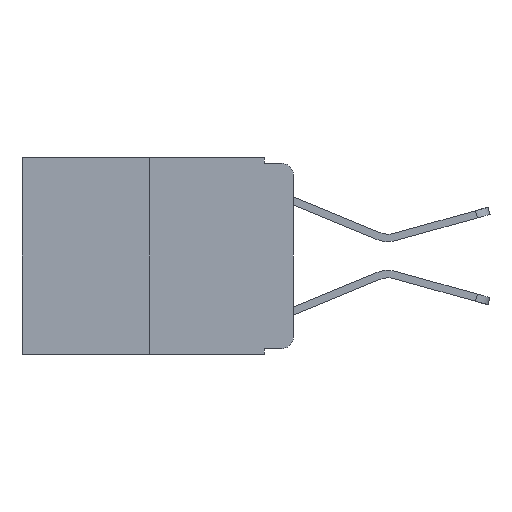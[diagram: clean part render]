
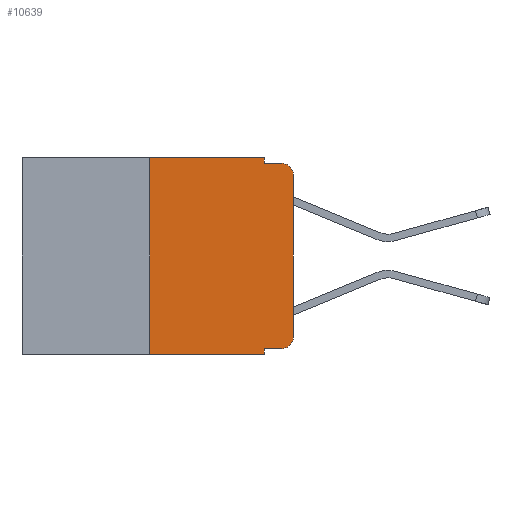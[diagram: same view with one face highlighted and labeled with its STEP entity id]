
A CAD part, left-side view. The second image highlights one B-rep face of the part: STEP entity #10639.
In plain terms, the highlighted planar face has unit normal (-1, 0, 0).
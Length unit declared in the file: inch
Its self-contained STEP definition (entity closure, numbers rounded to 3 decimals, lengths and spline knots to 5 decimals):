
#393 = LINE ( 'NONE', #5756, #20992 ) ;
#685 = DIRECTION ( 'NONE',  ( -1., 0., 0. ) ) ;
#1173 = VERTEX_POINT ( 'NONE', #13284 ) ;
#1434 = CARTESIAN_POINT ( 'NONE',  ( 0., 0.473, -0.343 ) ) ;
#1468 = CARTESIAN_POINT ( 'NONE',  ( 0., 0.25, 0. ) ) ;
#1786 = EDGE_CURVE ( 'NONE', #17790, #16491, #21317, .T. ) ;
#2402 = ORIENTED_EDGE ( 'NONE', *, *, #21774, .F. ) ;
#2690 = EDGE_CURVE ( 'NONE', #3242, #16491, #19737, .T. ) ;
#2977 = EDGE_CURVE ( 'NONE', #11182, #22603, #17582, .T. ) ;
#3242 = VERTEX_POINT ( 'NONE', #4226 ) ;
#3394 = CARTESIAN_POINT ( 'NONE',  ( 0., 0.051, -0.333 ) ) ;
#3872 = VECTOR ( 'NONE', #18371, 39.37008 ) ;
#4160 = AXIS2_PLACEMENT_3D ( 'NONE', #11089, #24662, #13111 ) ;
#4226 = CARTESIAN_POINT ( 'NONE',  ( 0., 0.25, -0.343 ) ) ;
#4704 = ORIENTED_EDGE ( 'NONE', *, *, #12614, .F. ) ;
#4867 = VECTOR ( 'NONE', #12065, 39.37008 ) ;
#4975 = CARTESIAN_POINT ( 'NONE',  ( 0., 0.473, 0. ) ) ;
#5521 = VERTEX_POINT ( 'NONE', #20653 ) ;
#5756 = CARTESIAN_POINT ( 'NONE',  ( 0., 0.051, -0.01 ) ) ;
#5895 = EDGE_CURVE ( 'NONE', #17790, #1173, #25040, .T. ) ;
#5953 = CARTESIAN_POINT ( 'NONE',  ( 0., 0.051, 0. ) ) ;
#6252 = DIRECTION ( 'NONE',  ( 0., -1., 0. ) ) ;
#6632 = EDGE_LOOP ( 'NONE', ( #18409, #18120, #2402, #21161, #15987, #4704, #15985, #20039, #12877, #23218 ) ) ;
#8086 = EDGE_CURVE ( 'NONE', #5521, #17999, #16842, .T. ) ;
#8513 = FACE_OUTER_BOUND ( 'NONE', #6632, .T. ) ;
#9139 = PLANE ( 'NONE',  #23047 ) ;
#9425 = CARTESIAN_POINT ( 'NONE',  ( 0., 0.051, -0.333 ) ) ;
#9535 = VECTOR ( 'NONE', #11433, 39.37008 ) ;
#9882 = DIRECTION ( 'NONE',  ( 0., -1., 0. ) ) ;
#9940 = EDGE_CURVE ( 'NONE', #17999, #14084, #13562, .T. ) ;
#10024 = CARTESIAN_POINT ( 'NONE',  ( 0., 0.051, -0.343 ) ) ;
#10639 = ADVANCED_FACE ( 'NONE', ( #8513 ), #9139, .F. ) ;
#11089 = CARTESIAN_POINT ( 'NONE',  ( 0., 0.02, -0.03 ) ) ;
#11144 = DIRECTION ( 'NONE',  ( 0., 0., -1. ) ) ;
#11182 = VERTEX_POINT ( 'NONE', #24507 ) ;
#11343 = VERTEX_POINT ( 'NONE', #1468 ) ;
#11433 = DIRECTION ( 'NONE',  ( 0., -1., 0. ) ) ;
#11603 = VECTOR ( 'NONE', #24381, 39.37008 ) ;
#11853 = VECTOR ( 'NONE', #14401, 39.37008 ) ;
#12065 = DIRECTION ( 'NONE',  ( 0., 0., -1. ) ) ;
#12128 = EDGE_CURVE ( 'NONE', #1173, #5521, #20756, .T. ) ;
#12212 = CARTESIAN_POINT ( 'NONE',  ( 0., 0., -0.03 ) ) ;
#12381 = VECTOR ( 'NONE', #13945, 39.37008 ) ;
#12614 = EDGE_CURVE ( 'NONE', #3242, #11343, #17082, .T. ) ;
#12788 = CARTESIAN_POINT ( 'NONE',  ( 0., 0.02, -0.313 ) ) ;
#12877 = ORIENTED_EDGE ( 'NONE', *, *, #5895, .T. ) ;
#13111 = DIRECTION ( 'NONE',  ( 0., 0., -1. ) ) ;
#13284 = CARTESIAN_POINT ( 'NONE',  ( 0., 0.02, -0.333 ) ) ;
#13562 = CIRCLE ( 'NONE', #4160, 0.02 ) ;
#13597 = CARTESIAN_POINT ( 'NONE',  ( 0., 0.051, 0. ) ) ;
#13945 = DIRECTION ( 'NONE',  ( 0., 0., -1. ) ) ;
#14084 = VERTEX_POINT ( 'NONE', #15018 ) ;
#14191 = CARTESIAN_POINT ( 'NONE',  ( 0., 0.051, -0.01 ) ) ;
#14401 = DIRECTION ( 'NONE',  ( 0., 0., 1. ) ) ;
#14766 = DIRECTION ( 'NONE',  ( 0., 0., -1. ) ) ;
#14778 = CARTESIAN_POINT ( 'NONE',  ( 0., 0., 0. ) ) ;
#15018 = CARTESIAN_POINT ( 'NONE',  ( 0., 0.02, -0.01 ) ) ;
#15985 = ORIENTED_EDGE ( 'NONE', *, *, #2690, .T. ) ;
#15987 = ORIENTED_EDGE ( 'NONE', *, *, #18081, .F. ) ;
#16491 = VERTEX_POINT ( 'NONE', #10024 ) ;
#16842 = LINE ( 'NONE', #14778, #11603 ) ;
#17082 = LINE ( 'NONE', #22136, #11853 ) ;
#17582 = LINE ( 'NONE', #13597, #12381 ) ;
#17790 = VERTEX_POINT ( 'NONE', #3394 ) ;
#17999 = VERTEX_POINT ( 'NONE', #12212 ) ;
#18056 = AXIS2_PLACEMENT_3D ( 'NONE', #12788, #685, #14766 ) ;
#18081 = EDGE_CURVE ( 'NONE', #11343, #11182, #19746, .T. ) ;
#18120 = ORIENTED_EDGE ( 'NONE', *, *, #9940, .T. ) ;
#18371 = DIRECTION ( 'NONE',  ( 0., -1., 0. ) ) ;
#18409 = ORIENTED_EDGE ( 'NONE', *, *, #8086, .T. ) ;
#19737 = LINE ( 'NONE', #1434, #23034 ) ;
#19746 = LINE ( 'NONE', #20229, #3872 ) ;
#20039 = ORIENTED_EDGE ( 'NONE', *, *, #1786, .F. ) ;
#20229 = CARTESIAN_POINT ( 'NONE',  ( 0., 0.473, 0. ) ) ;
#20653 = CARTESIAN_POINT ( 'NONE',  ( 0., 0., -0.313 ) ) ;
#20756 = CIRCLE ( 'NONE', #18056, 0.02 ) ;
#20992 = VECTOR ( 'NONE', #9882, 39.37008 ) ;
#21161 = ORIENTED_EDGE ( 'NONE', *, *, #2977, .F. ) ;
#21317 = LINE ( 'NONE', #5953, #4867 ) ;
#21774 = EDGE_CURVE ( 'NONE', #22603, #14084, #393, .T. ) ;
#22136 = CARTESIAN_POINT ( 'NONE',  ( 0., 0.25, 0. ) ) ;
#22603 = VERTEX_POINT ( 'NONE', #14191 ) ;
#22845 = DIRECTION ( 'NONE',  ( 1., 0., 0. ) ) ;
#23034 = VECTOR ( 'NONE', #6252, 39.37008 ) ;
#23047 = AXIS2_PLACEMENT_3D ( 'NONE', #4975, #22845, #11144 ) ;
#23218 = ORIENTED_EDGE ( 'NONE', *, *, #12128, .T. ) ;
#24381 = DIRECTION ( 'NONE',  ( 0., 0., 1. ) ) ;
#24507 = CARTESIAN_POINT ( 'NONE',  ( 0., 0.051, 0. ) ) ;
#24662 = DIRECTION ( 'NONE',  ( -1., 0., 0. ) ) ;
#25040 = LINE ( 'NONE', #9425, #9535 ) ;
